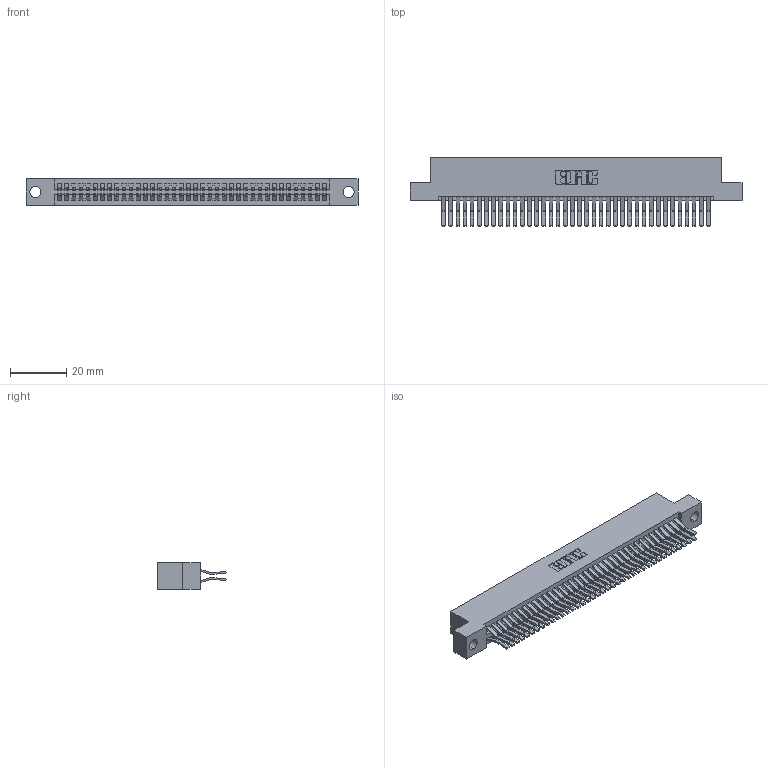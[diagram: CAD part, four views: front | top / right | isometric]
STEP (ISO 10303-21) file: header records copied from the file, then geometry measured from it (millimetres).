
FILE_DESCRIPTION (( 'STEP AP203' ), '1' );
FILE_NAME ('345-076-560-204.STEP', '2021-05-20T10:25:40', ( '' ), ( '' ), 'SwSTEP 2.0', 'SolidWorks 2020', '' );
FILE_SCHEMA (( 'CONFIG_CONTROL_DESIGN' ));
Length unit declared in the file: inch
Products named in the file (3): 345-292-001_560 Tail; 345-076-560-204; 345 Part_Flush Mounting Lugs - 0.156 Dia-TI
Assembly tree (77 placements, depth 2):
  345-076-560-204
    345 Part_Flush Mounting Lugs - 0.156 Dia-TI
    345-292-001_560 Tail  x76
Bounding box: 117.73 x 24.45 x 9.4 mm (x, y, z)
Volume: 11791.4 mm3; surface area: 18485 mm2
Topology: 77 solids, 77 shells, 4092 faces, 12157 edges, 8002 vertices
Faces by surface type: plane 2602, cylinder 1490
Entity records: 30861 total; most frequent: CARTESIAN_POINT 5182, ORIENTED_EDGE 5114, DIRECTION 4577, EDGE_CURVE 2557, VECTOR 2269, LINE 2269, VERTEX_POINT 1702, AXIS2_PLACEMENT_3D 1154
